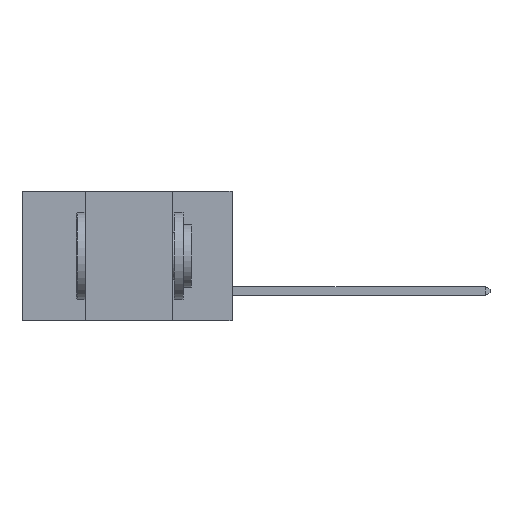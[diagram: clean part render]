
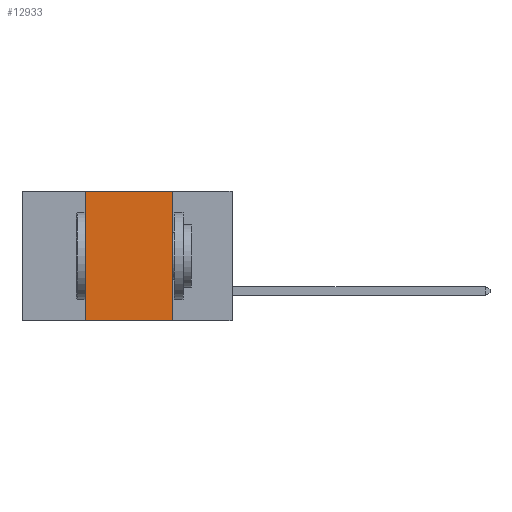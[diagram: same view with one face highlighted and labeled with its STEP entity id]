
A CAD part, left-side view. The second image highlights one B-rep face of the part: STEP entity #12933.
In plain terms, the highlighted planar face has unit normal (-1, 0, 0).
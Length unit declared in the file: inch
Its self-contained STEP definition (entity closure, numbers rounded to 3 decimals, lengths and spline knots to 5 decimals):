
#851 = VECTOR ( 'NONE', #31816, 39.37008 ) ;
#952 = CARTESIAN_POINT ( 'NONE',  ( 0., 0.6, 0. ) ) ;
#1041 = VERTEX_POINT ( 'NONE', #15322 ) ;
#2054 = EDGE_LOOP ( 'NONE', ( #22690, #22785, #22983, #23082 ) ) ;
#2810 = DIRECTION ( 'NONE',  ( 0., -1., 0. ) ) ;
#3520 = PLANE ( 'NONE',  #10218 ) ;
#3681 = EDGE_CURVE ( 'NONE', #16217, #30750, #9844, .T. ) ;
#4186 = CARTESIAN_POINT ( 'NONE',  ( 0., 0.42, 0. ) ) ;
#4299 = DIRECTION ( 'NONE',  ( 0., 0., 1. ) ) ;
#8578 = DIRECTION ( 'NONE',  ( 0., 0., -1. ) ) ;
#9079 = VECTOR ( 'NONE', #4299, 39.37008 ) ;
#9844 = LINE ( 'NONE', #4186, #9079 ) ;
#10145 = CARTESIAN_POINT ( 'NONE',  ( 0., 0.17, 0. ) ) ;
#10218 = AXIS2_PLACEMENT_3D ( 'NONE', #952, #23377, #8578 ) ;
#10380 = CARTESIAN_POINT ( 'NONE',  ( 0., 0.6, -0.37 ) ) ;
#10844 = FACE_OUTER_BOUND ( 'NONE', #2054, .T. ) ;
#11417 = LINE ( 'NONE', #10380, #17182 ) ;
#12592 = VECTOR ( 'NONE', #14999, 39.37008 ) ;
#12933 = ADVANCED_FACE ( 'NONE', ( #10844 ), #3520, .F. ) ;
#13173 = VERTEX_POINT ( 'NONE', #29156 ) ;
#14999 = DIRECTION ( 'NONE',  ( 0., 0., -1. ) ) ;
#15322 = CARTESIAN_POINT ( 'NONE',  ( 0., 0.17, 0. ) ) ;
#16217 = VERTEX_POINT ( 'NONE', #20477 ) ;
#17182 = VECTOR ( 'NONE', #2810, 39.37008 ) ;
#18868 = EDGE_CURVE ( 'NONE', #16217, #13173, #11417, .T. ) ;
#19942 = LINE ( 'NONE', #29338, #851 ) ;
#20477 = CARTESIAN_POINT ( 'NONE',  ( 0., 0.42, -0.37 ) ) ;
#22690 = ORIENTED_EDGE ( 'NONE', *, *, #31297, .F. ) ;
#22785 = ORIENTED_EDGE ( 'NONE', *, *, #27886, .F. ) ;
#22983 = ORIENTED_EDGE ( 'NONE', *, *, #3681, .F. ) ;
#23082 = ORIENTED_EDGE ( 'NONE', *, *, #18868, .T. ) ;
#23377 = DIRECTION ( 'NONE',  ( 1., 0., 0. ) ) ;
#25701 = LINE ( 'NONE', #10145, #12592 ) ;
#27886 = EDGE_CURVE ( 'NONE', #30750, #1041, #19942, .T. ) ;
#29156 = CARTESIAN_POINT ( 'NONE',  ( 0., 0.17, -0.37 ) ) ;
#29338 = CARTESIAN_POINT ( 'NONE',  ( 0., 0.6, 0. ) ) ;
#30132 = CARTESIAN_POINT ( 'NONE',  ( 0., 0.42, 0. ) ) ;
#30750 = VERTEX_POINT ( 'NONE', #30132 ) ;
#31297 = EDGE_CURVE ( 'NONE', #1041, #13173, #25701, .T. ) ;
#31816 = DIRECTION ( 'NONE',  ( 0., -1., 0. ) ) ;
